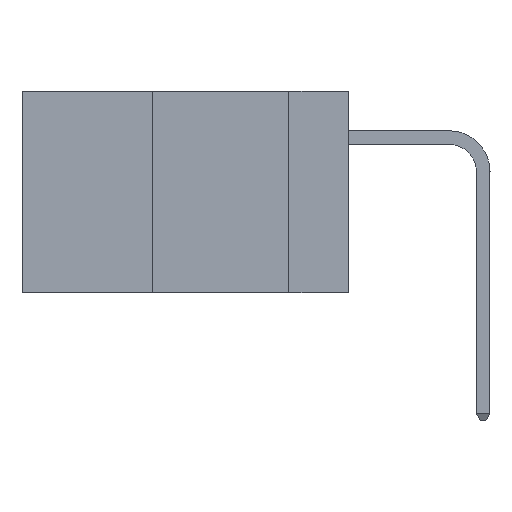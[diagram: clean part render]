
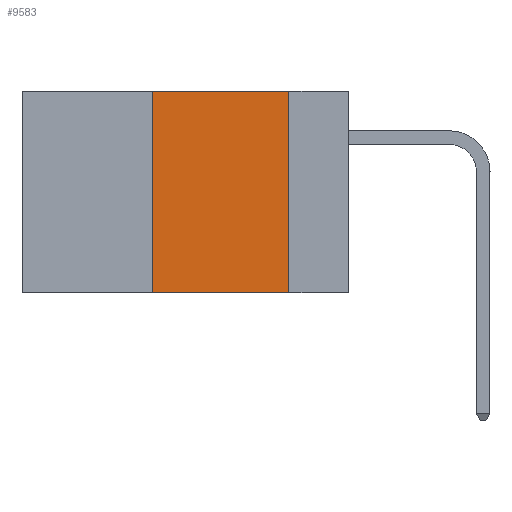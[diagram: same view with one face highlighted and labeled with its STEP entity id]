
A CAD part, left-side view. The second image highlights one B-rep face of the part: STEP entity #9583.
In plain terms, the highlighted planar face has unit normal (-1, 0, 0).
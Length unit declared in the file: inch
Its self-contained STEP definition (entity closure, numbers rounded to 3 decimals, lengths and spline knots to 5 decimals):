
#138 = VECTOR ( 'NONE', #16421, 39.37008 ) ;
#2799 = EDGE_CURVE ( 'NONE', #6277, #20875, #7961, .T. ) ;
#3127 = ORIENTED_EDGE ( 'NONE', *, *, #20061, .F. ) ;
#3775 = VERTEX_POINT ( 'NONE', #4805 ) ;
#4027 = CARTESIAN_POINT ( 'NONE',  ( 0., 0.6, -0.37 ) ) ;
#4418 = EDGE_CURVE ( 'NONE', #8597, #3775, #15256, .T. ) ;
#4431 = CARTESIAN_POINT ( 'NONE',  ( 0., 0.6, 0. ) ) ;
#4805 = CARTESIAN_POINT ( 'NONE',  ( 0., 0.11, 0. ) ) ;
#5760 = CARTESIAN_POINT ( 'NONE',  ( 0., 0.36, -0.37 ) ) ;
#6277 = VERTEX_POINT ( 'NONE', #5760 ) ;
#7601 = LINE ( 'NONE', #15186, #12573 ) ;
#7961 = LINE ( 'NONE', #4027, #12368 ) ;
#8104 = LINE ( 'NONE', #9334, #12513 ) ;
#8146 = DIRECTION ( 'NONE',  ( 1., 0., 0. ) ) ;
#8597 = VERTEX_POINT ( 'NONE', #21992 ) ;
#8659 = ORIENTED_EDGE ( 'NONE', *, *, #4418, .F. ) ;
#9334 = CARTESIAN_POINT ( 'NONE',  ( 0., 0.36, 0. ) ) ;
#9534 = DIRECTION ( 'NONE',  ( 0., 0., -1. ) ) ;
#9583 = ADVANCED_FACE ( 'NONE', ( #12390 ), #15646, .F. ) ;
#9584 = DIRECTION ( 'NONE',  ( 0., -1., 0. ) ) ;
#11018 = ORIENTED_EDGE ( 'NONE', *, *, #2799, .T. ) ;
#11206 = DIRECTION ( 'NONE',  ( 0., 0., 1. ) ) ;
#12368 = VECTOR ( 'NONE', #9584, 39.37008 ) ;
#12390 = FACE_OUTER_BOUND ( 'NONE', #17786, .T. ) ;
#12513 = VECTOR ( 'NONE', #11206, 39.37008 ) ;
#12573 = VECTOR ( 'NONE', #9534, 39.37008 ) ;
#14219 = EDGE_CURVE ( 'NONE', #6277, #8597, #8104, .T. ) ;
#15186 = CARTESIAN_POINT ( 'NONE',  ( 0., 0.11, 0. ) ) ;
#15256 = LINE ( 'NONE', #23798, #138 ) ;
#15646 = PLANE ( 'NONE',  #21192 ) ;
#16421 = DIRECTION ( 'NONE',  ( 0., -1., 0. ) ) ;
#17293 = CARTESIAN_POINT ( 'NONE',  ( 0., 0.11, -0.37 ) ) ;
#17786 = EDGE_LOOP ( 'NONE', ( #3127, #8659, #23042, #11018 ) ) ;
#20061 = EDGE_CURVE ( 'NONE', #3775, #20875, #7601, .T. ) ;
#20875 = VERTEX_POINT ( 'NONE', #17293 ) ;
#21192 = AXIS2_PLACEMENT_3D ( 'NONE', #4431, #8146, #21286 ) ;
#21286 = DIRECTION ( 'NONE',  ( 0., 0., -1. ) ) ;
#21992 = CARTESIAN_POINT ( 'NONE',  ( 0., 0.36, 0. ) ) ;
#23042 = ORIENTED_EDGE ( 'NONE', *, *, #14219, .F. ) ;
#23798 = CARTESIAN_POINT ( 'NONE',  ( 0., 0.6, 0. ) ) ;
